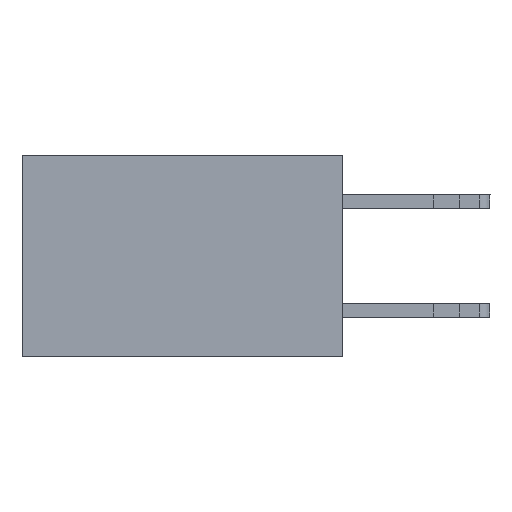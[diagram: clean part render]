
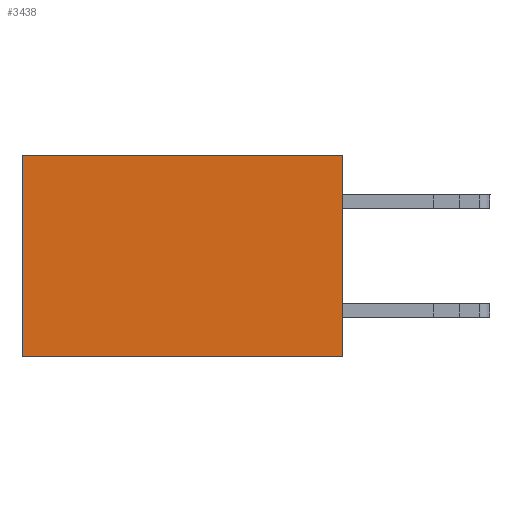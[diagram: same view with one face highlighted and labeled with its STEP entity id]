
A CAD part, left-side view. The second image highlights one B-rep face of the part: STEP entity #3438.
In plain terms, the highlighted planar face has unit normal (-1, 0, 0).
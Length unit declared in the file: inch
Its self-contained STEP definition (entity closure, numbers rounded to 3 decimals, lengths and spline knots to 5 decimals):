
#33 = EDGE_CURVE ( 'NONE', #13248, #128, #28292, .T. ) ;
#128 = VERTEX_POINT ( 'NONE', #11429 ) ;
#450 = EDGE_LOOP ( 'NONE', ( #28178, #3236, #9696, #3544 ) ) ;
#832 = DIRECTION ( 'NONE',  ( 0., 0., -1. ) ) ;
#1100 = CARTESIAN_POINT ( 'NONE',  ( 0.277, 0.59, 0. ) ) ;
#2176 = DIRECTION ( 'NONE',  ( 0., 1., 0. ) ) ;
#3236 = ORIENTED_EDGE ( 'NONE', *, *, #13858, .F. ) ;
#3419 = PLANE ( 'NONE',  #16915 ) ;
#3438 = ADVANCED_FACE ( 'NONE', ( #27978 ), #3419, .F. ) ;
#3544 = ORIENTED_EDGE ( 'NONE', *, *, #21451, .T. ) ;
#5507 = DIRECTION ( 'NONE',  ( 1., 0., 0. ) ) ;
#5905 = VERTEX_POINT ( 'NONE', #16162 ) ;
#6514 = LINE ( 'NONE', #31404, #27519 ) ;
#7207 = LINE ( 'NONE', #19418, #25383 ) ;
#8925 = VECTOR ( 'NONE', #27397, 39.37008 ) ;
#9696 = ORIENTED_EDGE ( 'NONE', *, *, #10029, .F. ) ;
#10029 = EDGE_CURVE ( 'NONE', #5905, #25031, #17604, .T. ) ;
#10517 = VECTOR ( 'NONE', #832, 39.37008 ) ;
#11429 = CARTESIAN_POINT ( 'NONE',  ( 0.277, 0.59, -0.37 ) ) ;
#13047 = DIRECTION ( 'NONE',  ( 0., 0., -1. ) ) ;
#13248 = VERTEX_POINT ( 'NONE', #1100 ) ;
#13697 = CARTESIAN_POINT ( 'NONE',  ( 0.277, 0.59, -0.37 ) ) ;
#13858 = EDGE_CURVE ( 'NONE', #25031, #128, #6514, .T. ) ;
#16162 = CARTESIAN_POINT ( 'NONE',  ( 0.277, 0., 0. ) ) ;
#16915 = AXIS2_PLACEMENT_3D ( 'NONE', #20735, #5507, #13047 ) ;
#17604 = LINE ( 'NONE', #25294, #8925 ) ;
#19418 = CARTESIAN_POINT ( 'NONE',  ( 0.277, 0., 0. ) ) ;
#19792 = CARTESIAN_POINT ( 'NONE',  ( 0.277, 0., -0.37 ) ) ;
#19884 = DIRECTION ( 'NONE',  ( 0., 1., 0. ) ) ;
#20735 = CARTESIAN_POINT ( 'NONE',  ( 0.277, 0., -0.37 ) ) ;
#21451 = EDGE_CURVE ( 'NONE', #5905, #13248, #7207, .T. ) ;
#25031 = VERTEX_POINT ( 'NONE', #19792 ) ;
#25294 = CARTESIAN_POINT ( 'NONE',  ( 0.277, 0., -0.37 ) ) ;
#25383 = VECTOR ( 'NONE', #19884, 39.37008 ) ;
#27397 = DIRECTION ( 'NONE',  ( 0., 0., -1. ) ) ;
#27519 = VECTOR ( 'NONE', #2176, 39.37008 ) ;
#27978 = FACE_OUTER_BOUND ( 'NONE', #450, .T. ) ;
#28178 = ORIENTED_EDGE ( 'NONE', *, *, #33, .T. ) ;
#28292 = LINE ( 'NONE', #13697, #10517 ) ;
#31404 = CARTESIAN_POINT ( 'NONE',  ( 0.277, 0., -0.37 ) ) ;
